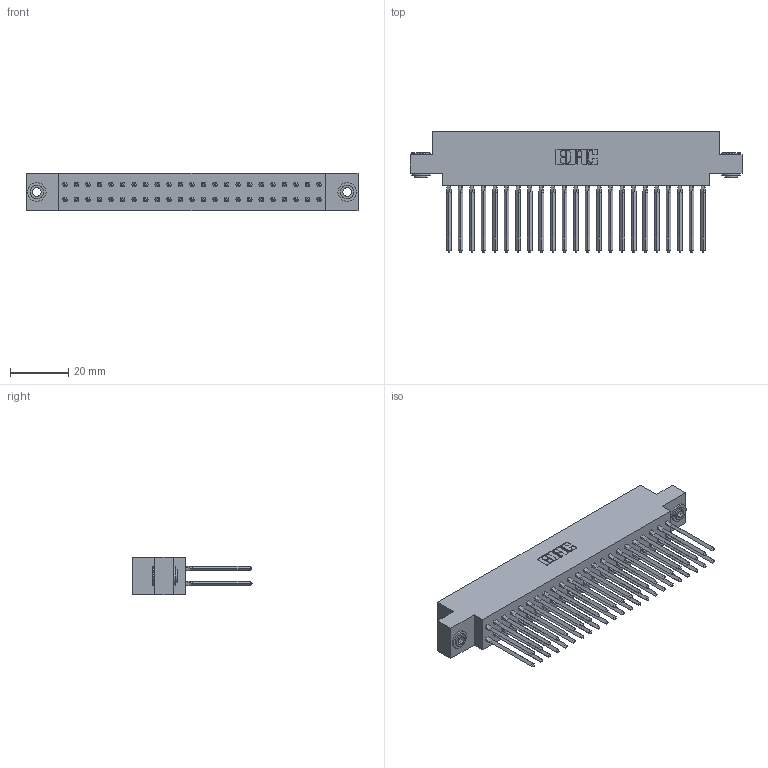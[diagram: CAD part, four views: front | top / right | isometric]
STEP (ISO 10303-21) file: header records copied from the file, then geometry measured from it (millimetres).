
FILE_DESCRIPTION (( 'STEP AP203' ), '1' );
FILE_NAME ('317-046-543-803.STEP', '2020-02-28T02:34:22', ( '' ), ( '' ), 'SwSTEP 2.0', 'SolidWorks 2016', '' );
FILE_SCHEMA (( 'CONFIG_CONTROL_DESIGN' ));
Length unit declared in the file: inch
Products named in the file (4): 317-046-543-803; 345-250-002_345-250-002-102; 317-290-001_543; 317 Part_.156 Dia - TH
Assembly tree (49 placements, depth 2):
  317-046-543-803
    317 Part_.156 Dia - TH
    317-290-001_543  x46
    345-250-002_345-250-002-102  x2
Bounding box: 113.84 x 41.15 x 12.7 mm (x, y, z)
Volume: 18712.3 mm3; surface area: 27853.9 mm2
Topology: 49 solids, 49 shells, 4234 faces, 11713 edges, 7544 vertices
Faces by surface type: plane 3426, cylinder 616, bspline 184, cone 8
Entity records: 36547 total; most frequent: CARTESIAN_POINT 6758, ORIENTED_EDGE 6250, DIRECTION 5257, EDGE_CURVE 3125, VECTOR 2845, LINE 2845, VERTEX_POINT 2075, AXIS2_PLACEMENT_3D 1206
